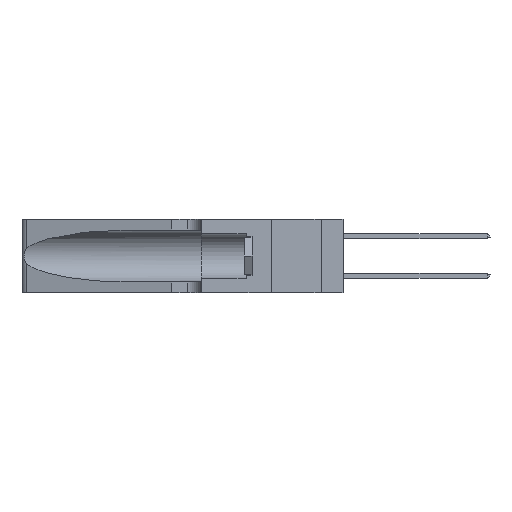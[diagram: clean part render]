
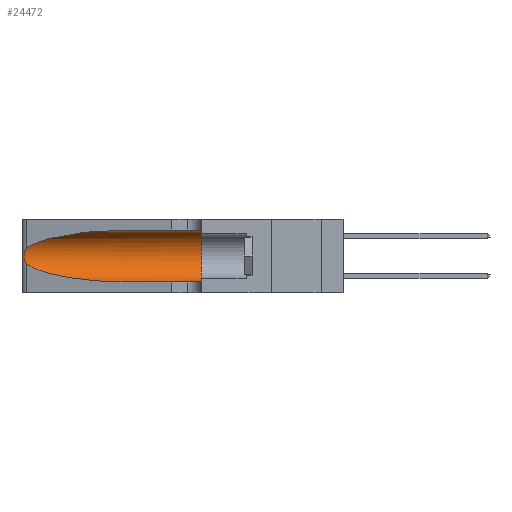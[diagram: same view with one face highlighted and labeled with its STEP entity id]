
A CAD part, left-side view. The second image highlights one B-rep face of the part: STEP entity #24472.
In plain terms, the highlighted cylindrical face has radius 3.308 mm (diameter 6.617 mm), a partial arc.
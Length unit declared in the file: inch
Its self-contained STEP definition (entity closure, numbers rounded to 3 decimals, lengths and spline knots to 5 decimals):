
#953 = CARTESIAN_POINT ( 'NONE',  ( 0.1305, 0.35, 0.31525 ) ) ;
#1115 =( BOUNDED_CURVE ( )  B_SPLINE_CURVE ( 3, ( #29830, #18531, #20827, #6929 ),
 .UNSPECIFIED., .F., .F. ) 
 B_SPLINE_CURVE_WITH_KNOTS ( ( 4, 4 ),
 ( 3.44316, 4.71239 ),
 .UNSPECIFIED. ) 
 CURVE ( )  GEOMETRIC_REPRESENTATION_ITEM ( )  RATIONAL_B_SPLINE_CURVE ( ( 1., 0.87, 0.87, 1. ) ) 
 REPRESENTATION_ITEM ( '' )  );
#1151 =( BOUNDED_CURVE ( )  B_SPLINE_CURVE ( 3, ( #29929, #13887, #18535, #4534 ),
 .UNSPECIFIED., .F., .F. ) 
 B_SPLINE_CURVE_WITH_KNOTS ( ( 4, 4 ),
 ( 1.5708, 2.84003 ),
 .UNSPECIFIED. ) 
 CURVE ( )  GEOMETRIC_REPRESENTATION_ITEM ( )  RATIONAL_B_SPLINE_CURVE ( ( 1., 0.87, 0.87, 1. ) ) 
 REPRESENTATION_ITEM ( '' )  );
#1292 = DIRECTION ( 'NONE',  ( 0., -1., 0. ) ) ;
#1630 = CARTESIAN_POINT ( 'NONE',  ( 0.25555, 1.22994, 0.2215 ) ) ;
#1859 = LINE ( 'NONE', #28105, #3360 ) ;
#2090 = B_SPLINE_CURVE_WITH_KNOTS ( 'NONE', 3,
 ( #13380, #1630, #18021, #4014, #20319, #6421, #22625, #8841, #24914, #11189, #27240, #13484, #29528, #15799 ),
 .UNSPECIFIED., .F., .F.,
 ( 4, 2, 2, 2, 2, 2, 4 ),
 ( 0., 0.00027, 0.00053, 0.00107, 0.0016, 0.00187, 0.00214 ),
 .UNSPECIFIED. ) ;
#2481 = EDGE_CURVE ( 'NONE', #4720, #20328, #28368, .T. ) ;
#3129 = CARTESIAN_POINT ( 'NONE',  ( 0.1305, 0.72297, 0.31525 ) ) ;
#3360 = VECTOR ( 'NONE', #14354, 39.37008 ) ;
#3502 = AXIS2_PLACEMENT_3D ( 'NONE', #10585, #17523, #5796 ) ;
#4014 = CARTESIAN_POINT ( 'NONE',  ( 0.25787, 1.23484, 0.2124 ) ) ;
#4534 = CARTESIAN_POINT ( 'NONE',  ( 0.25487, 1.22718, 0.22369 ) ) ;
#4586 = DIRECTION ( 'NONE',  ( 0., 1., 0. ) ) ;
#4720 = VERTEX_POINT ( 'NONE', #953 ) ;
#5796 = DIRECTION ( 'NONE',  ( 0., 0., -1. ) ) ;
#6178 = VERTEX_POINT ( 'NONE', #6338 ) ;
#6299 = EDGE_LOOP ( 'NONE', ( #10908, #7093, #11777, #28321, #7619, #24050 ) ) ;
#6322 = AXIS2_PLACEMENT_3D ( 'NONE', #18585, #4586, #20878 ) ;
#6338 = CARTESIAN_POINT ( 'NONE',  ( 0.25487, 1.22718, 0.22369 ) ) ;
#6421 = CARTESIAN_POINT ( 'NONE',  ( 0.26018, 1.23835, 0.19895 ) ) ;
#6929 = CARTESIAN_POINT ( 'NONE',  ( 0.1305, 0.72297, 0.05475 ) ) ;
#7093 = ORIENTED_EDGE ( 'NONE', *, *, #11393, .T. ) ;
#7619 = ORIENTED_EDGE ( 'NONE', *, *, #2481, .F. ) ;
#8841 = CARTESIAN_POINT ( 'NONE',  ( 0.26075, 1.23896, 0.178 ) ) ;
#9416 = VERTEX_POINT ( 'NONE', #24884 ) ;
#9575 = LINE ( 'NONE', #24482, #14257 ) ;
#10585 = CARTESIAN_POINT ( 'NONE',  ( 0.1305, 1.61858, 0.185 ) ) ;
#10908 = ORIENTED_EDGE ( 'NONE', *, *, #14512, .T. ) ;
#11189 = CARTESIAN_POINT ( 'NONE',  ( 0.25856, 1.23593, 0.16098 ) ) ;
#11393 = EDGE_CURVE ( 'NONE', #6178, #24654, #2090, .T. ) ;
#11777 = ORIENTED_EDGE ( 'NONE', *, *, #13437, .T. ) ;
#11964 = EDGE_CURVE ( 'NONE', #9416, #20328, #9575, .T. ) ;
#13380 = CARTESIAN_POINT ( 'NONE',  ( 0.25487, 1.22718, 0.22369 ) ) ;
#13437 = EDGE_CURVE ( 'NONE', #24654, #9416, #1115, .T. ) ;
#13484 = CARTESIAN_POINT ( 'NONE',  ( 0.25639, 1.23186, 0.15144 ) ) ;
#13887 = CARTESIAN_POINT ( 'NONE',  ( 0.18966, 0.96281, 0.31525 ) ) ;
#14257 = VECTOR ( 'NONE', #1292, 39.37008 ) ;
#14354 = DIRECTION ( 'NONE',  ( 0., -1., 0. ) ) ;
#14512 = EDGE_CURVE ( 'NONE', #29718, #6178, #1151, .T. ) ;
#15427 = FACE_OUTER_BOUND ( 'NONE', #6299, .T. ) ;
#15799 = CARTESIAN_POINT ( 'NONE',  ( 0.25487, 1.22718, 0.14631 ) ) ;
#17523 = DIRECTION ( 'NONE',  ( 0., -1., 0. ) ) ;
#18021 = CARTESIAN_POINT ( 'NONE',  ( 0.25639, 1.23184, 0.21858 ) ) ;
#18531 = CARTESIAN_POINT ( 'NONE',  ( 0.2373, 1.15595, 0.08982 ) ) ;
#18535 = CARTESIAN_POINT ( 'NONE',  ( 0.2373, 1.15595, 0.28018 ) ) ;
#18585 = CARTESIAN_POINT ( 'NONE',  ( 0.1305, 0.35, 0.185 ) ) ;
#18710 = EDGE_CURVE ( 'NONE', #29718, #4720, #1859, .T. ) ;
#20319 = CARTESIAN_POINT ( 'NONE',  ( 0.25854, 1.2359, 0.20912 ) ) ;
#20328 = VERTEX_POINT ( 'NONE', #24898 ) ;
#20827 = CARTESIAN_POINT ( 'NONE',  ( 0.18966, 0.96281, 0.05475 ) ) ;
#20830 = CYLINDRICAL_SURFACE ( 'NONE', #3502, 0.13025 ) ;
#20878 = DIRECTION ( 'NONE',  ( 0., 0., 1. ) ) ;
#22618 = CARTESIAN_POINT ( 'NONE',  ( 0.25487, 1.22718, 0.14631 ) ) ;
#22625 = CARTESIAN_POINT ( 'NONE',  ( 0.26075, 1.23896, 0.19203 ) ) ;
#24050 = ORIENTED_EDGE ( 'NONE', *, *, #18710, .F. ) ;
#24472 = ADVANCED_FACE ( 'NONE', ( #15427 ), #20830, .F. ) ;
#24482 = CARTESIAN_POINT ( 'NONE',  ( 0.1305, 1.61858, 0.05475 ) ) ;
#24654 = VERTEX_POINT ( 'NONE', #22618 ) ;
#24884 = CARTESIAN_POINT ( 'NONE',  ( 0.1305, 0.72297, 0.05475 ) ) ;
#24898 = CARTESIAN_POINT ( 'NONE',  ( 0.1305, 0.35, 0.05475 ) ) ;
#24914 = CARTESIAN_POINT ( 'NONE',  ( 0.26017, 1.23833, 0.17102 ) ) ;
#27240 = CARTESIAN_POINT ( 'NONE',  ( 0.25789, 1.23486, 0.15765 ) ) ;
#28105 = CARTESIAN_POINT ( 'NONE',  ( 0.1305, 1.61858, 0.31525 ) ) ;
#28321 = ORIENTED_EDGE ( 'NONE', *, *, #11964, .T. ) ;
#28368 = CIRCLE ( 'NONE', #6322, 0.13025 ) ;
#29528 = CARTESIAN_POINT ( 'NONE',  ( 0.25555, 1.22993, 0.14849 ) ) ;
#29718 = VERTEX_POINT ( 'NONE', #3129 ) ;
#29830 = CARTESIAN_POINT ( 'NONE',  ( 0.25487, 1.22718, 0.14631 ) ) ;
#29929 = CARTESIAN_POINT ( 'NONE',  ( 0.1305, 0.72297, 0.31525 ) ) ;
